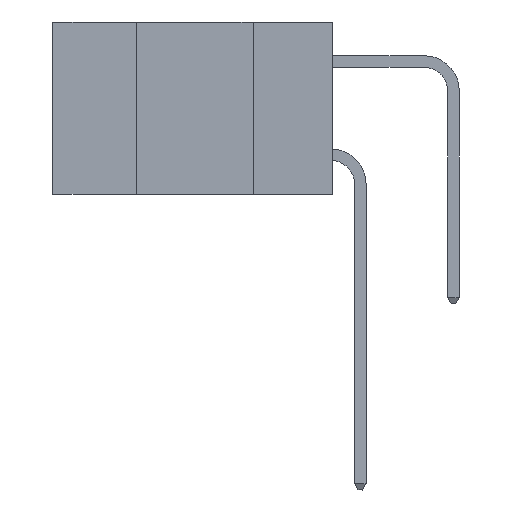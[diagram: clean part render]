
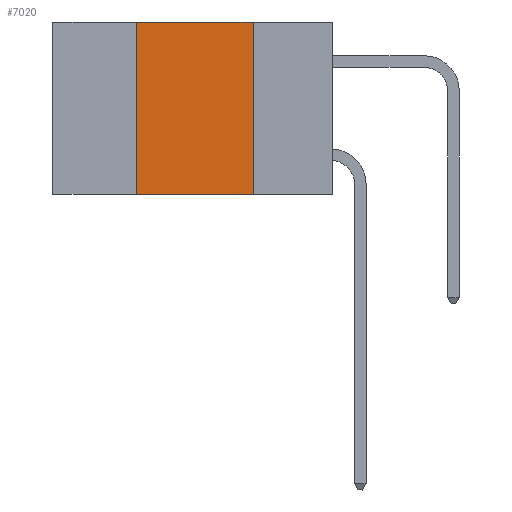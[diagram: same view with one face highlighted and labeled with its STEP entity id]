
A CAD part, left-side view. The second image highlights one B-rep face of the part: STEP entity #7020.
In plain terms, the highlighted planar face has unit normal (-1, 0, 0).
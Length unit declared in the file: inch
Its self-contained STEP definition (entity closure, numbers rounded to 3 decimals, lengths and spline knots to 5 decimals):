
#209 = VECTOR ( 'NONE', #6956, 39.37008 ) ;
#1447 = VERTEX_POINT ( 'NONE', #3663 ) ;
#2495 = ORIENTED_EDGE ( 'NONE', *, *, #20104, .F. ) ;
#2836 = FACE_OUTER_BOUND ( 'NONE', #11519, .T. ) ;
#3644 = CARTESIAN_POINT ( 'NONE',  ( 0., 0.17, 0. ) ) ;
#3663 = CARTESIAN_POINT ( 'NONE',  ( 0., 0.42, 0. ) ) ;
#4571 = EDGE_CURVE ( 'NONE', #1447, #9477, #14108, .T. ) ;
#5118 = VECTOR ( 'NONE', #13872, 39.37008 ) ;
#5485 = DIRECTION ( 'NONE',  ( 0., 0., 1. ) ) ;
#6044 = CARTESIAN_POINT ( 'NONE',  ( 0., 0.17, 0. ) ) ;
#6956 = DIRECTION ( 'NONE',  ( 0., 0., -1. ) ) ;
#7020 = ADVANCED_FACE ( 'NONE', ( #2836 ), #11163, .F. ) ;
#8388 = VECTOR ( 'NONE', #5485, 39.37008 ) ;
#8412 = AXIS2_PLACEMENT_3D ( 'NONE', #10923, #10569, #9418 ) ;
#9418 = DIRECTION ( 'NONE',  ( 0., 0., -1. ) ) ;
#9477 = VERTEX_POINT ( 'NONE', #6044 ) ;
#9539 = LINE ( 'NONE', #3644, #209 ) ;
#9820 = VERTEX_POINT ( 'NONE', #20039 ) ;
#9889 = VECTOR ( 'NONE', #15509, 39.37008 ) ;
#10403 = EDGE_CURVE ( 'NONE', #13917, #9820, #17914, .T. ) ;
#10569 = DIRECTION ( 'NONE',  ( 1., 0., 0. ) ) ;
#10923 = CARTESIAN_POINT ( 'NONE',  ( 0., 0.6, 0. ) ) ;
#11163 = PLANE ( 'NONE',  #8412 ) ;
#11519 = EDGE_LOOP ( 'NONE', ( #2495, #14779, #15952, #14602 ) ) ;
#11926 = CARTESIAN_POINT ( 'NONE',  ( 0., 0.42, 0. ) ) ;
#12171 = EDGE_CURVE ( 'NONE', #13917, #1447, #16860, .T. ) ;
#13872 = DIRECTION ( 'NONE',  ( 0., -1., 0. ) ) ;
#13917 = VERTEX_POINT ( 'NONE', #19694 ) ;
#14062 = CARTESIAN_POINT ( 'NONE',  ( 0., 0.6, -0.37 ) ) ;
#14108 = LINE ( 'NONE', #20179, #9889 ) ;
#14602 = ORIENTED_EDGE ( 'NONE', *, *, #10403, .T. ) ;
#14779 = ORIENTED_EDGE ( 'NONE', *, *, #4571, .F. ) ;
#15509 = DIRECTION ( 'NONE',  ( 0., -1., 0. ) ) ;
#15952 = ORIENTED_EDGE ( 'NONE', *, *, #12171, .F. ) ;
#16860 = LINE ( 'NONE', #11926, #8388 ) ;
#17914 = LINE ( 'NONE', #14062, #5118 ) ;
#19694 = CARTESIAN_POINT ( 'NONE',  ( 0., 0.42, -0.37 ) ) ;
#20039 = CARTESIAN_POINT ( 'NONE',  ( 0., 0.17, -0.37 ) ) ;
#20104 = EDGE_CURVE ( 'NONE', #9477, #9820, #9539, .T. ) ;
#20179 = CARTESIAN_POINT ( 'NONE',  ( 0., 0.6, 0. ) ) ;
